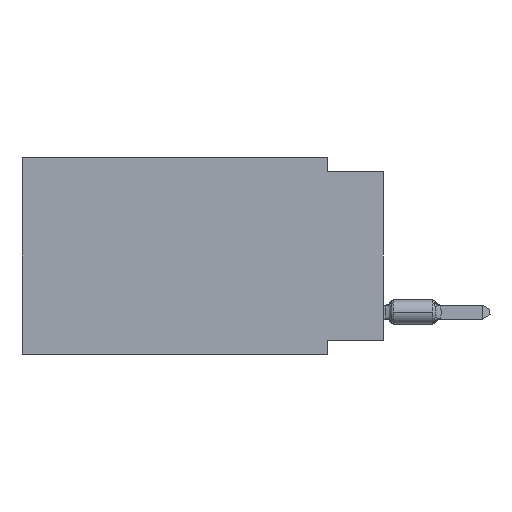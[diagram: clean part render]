
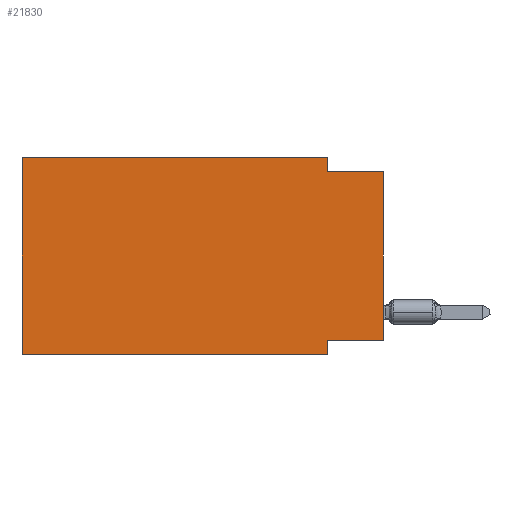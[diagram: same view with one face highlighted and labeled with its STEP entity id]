
A CAD part, left-side view. The second image highlights one B-rep face of the part: STEP entity #21830.
In plain terms, the highlighted planar face has unit normal (-1, 0, 0).
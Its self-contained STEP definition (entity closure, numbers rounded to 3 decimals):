
#452 = LINE ( 'NONE', #8074, #16340 ) ;
#2260 = EDGE_CURVE ( 'NONE', #10418, #6715, #41515, .T. ) ;
#3924 = VERTEX_POINT ( 'NONE', #22637 ) ;
#4079 = ORIENTED_EDGE ( 'NONE', *, *, #33845, .F. ) ;
#5084 = VECTOR ( 'NONE', #5566, 1000. ) ;
#5566 = DIRECTION ( 'NONE',  ( 0., 0., 1. ) ) ;
#6008 = VECTOR ( 'NONE', #10303, 1000. ) ;
#6026 = DIRECTION ( 'NONE',  ( 0., 0., -1. ) ) ;
#6108 = LINE ( 'NONE', #26974, #5084 ) ;
#6715 = VERTEX_POINT ( 'NONE', #27822 ) ;
#6781 = LINE ( 'NONE', #32423, #36512 ) ;
#7133 = ORIENTED_EDGE ( 'NONE', *, *, #13305, .F. ) ;
#8074 = CARTESIAN_POINT ( 'NONE',  ( 0., 16.383, 0. ) ) ;
#10226 = FACE_OUTER_BOUND ( 'NONE', #10283, .T. ) ;
#10283 = EDGE_LOOP ( 'NONE', ( #15879, #4079, #47292, #52221, #31678, #54057, #44423, #7133 ) ) ;
#10303 = DIRECTION ( 'NONE',  ( 0., 1., 0. ) ) ;
#10418 = VERTEX_POINT ( 'NONE', #30721 ) ;
#11754 = EDGE_CURVE ( 'NONE', #43430, #31384, #45235, .T. ) ;
#13175 = EDGE_CURVE ( 'NONE', #3924, #39061, #6108, .T. ) ;
#13305 = EDGE_CURVE ( 'NONE', #3924, #40642, #48945, .T. ) ;
#15879 = ORIENTED_EDGE ( 'NONE', *, *, #13175, .T. ) ;
#16051 = DIRECTION ( 'NONE',  ( 0., -1., 0. ) ) ;
#16340 = VECTOR ( 'NONE', #25536, 1000. ) ;
#16719 = CARTESIAN_POINT ( 'NONE',  ( 0., 2.54, 0. ) ) ;
#18103 = CARTESIAN_POINT ( 'NONE',  ( 0., 16.383, 0. ) ) ;
#18830 = EDGE_CURVE ( 'NONE', #10418, #54028, #452, .T. ) ;
#19998 = LINE ( 'NONE', #49879, #47652 ) ;
#21830 = ADVANCED_FACE ( 'NONE', ( #10226 ), #35350, .F. ) ;
#22637 = CARTESIAN_POINT ( 'NONE',  ( 0., 0., -8.255 ) ) ;
#25536 = DIRECTION ( 'NONE',  ( 0., 0., 1. ) ) ;
#25730 = DIRECTION ( 'NONE',  ( 0., 0., -1. ) ) ;
#26595 = DIRECTION ( 'NONE',  ( 1., 0., 0. ) ) ;
#26870 = VECTOR ( 'NONE', #32484, 1000. ) ;
#26974 = CARTESIAN_POINT ( 'NONE',  ( 0., 0., 0. ) ) ;
#27822 = CARTESIAN_POINT ( 'NONE',  ( 0., 2.54, -8.89 ) ) ;
#28041 = CARTESIAN_POINT ( 'NONE',  ( 0., 0., -0.635 ) ) ;
#30721 = CARTESIAN_POINT ( 'NONE',  ( 0., 16.383, -8.89 ) ) ;
#31384 = VERTEX_POINT ( 'NONE', #52134 ) ;
#31678 = ORIENTED_EDGE ( 'NONE', *, *, #18830, .F. ) ;
#32132 = DIRECTION ( 'NONE',  ( 0., 0., -1. ) ) ;
#32423 = CARTESIAN_POINT ( 'NONE',  ( 0., 2.54, -8.89 ) ) ;
#32484 = DIRECTION ( 'NONE',  ( 0., -1., 0. ) ) ;
#33845 = EDGE_CURVE ( 'NONE', #31384, #39061, #39145, .T. ) ;
#35350 = PLANE ( 'NONE',  #41763 ) ;
#36512 = VECTOR ( 'NONE', #32132, 1000. ) ;
#39061 = VERTEX_POINT ( 'NONE', #28041 ) ;
#39145 = LINE ( 'NONE', #55516, #47612 ) ;
#40512 = CARTESIAN_POINT ( 'NONE',  ( 0., 0., -8.255 ) ) ;
#40642 = VERTEX_POINT ( 'NONE', #41269 ) ;
#41269 = CARTESIAN_POINT ( 'NONE',  ( 0., 2.54, -8.255 ) ) ;
#41515 = LINE ( 'NONE', #53915, #26870 ) ;
#41763 = AXIS2_PLACEMENT_3D ( 'NONE', #53382, #26595, #6026 ) ;
#43430 = VERTEX_POINT ( 'NONE', #48754 ) ;
#44423 = ORIENTED_EDGE ( 'NONE', *, *, #50243, .F. ) ;
#45235 = LINE ( 'NONE', #16719, #45657 ) ;
#45657 = VECTOR ( 'NONE', #25730, 1000. ) ;
#47292 = ORIENTED_EDGE ( 'NONE', *, *, #11754, .F. ) ;
#47612 = VECTOR ( 'NONE', #47897, 1000. ) ;
#47652 = VECTOR ( 'NONE', #16051, 1000. ) ;
#47897 = DIRECTION ( 'NONE',  ( 0., -1., 0. ) ) ;
#48754 = CARTESIAN_POINT ( 'NONE',  ( 0., 2.54, 0. ) ) ;
#48945 = LINE ( 'NONE', #40512, #6008 ) ;
#49879 = CARTESIAN_POINT ( 'NONE',  ( 0., 16.383, 0. ) ) ;
#50243 = EDGE_CURVE ( 'NONE', #40642, #6715, #6781, .T. ) ;
#52134 = CARTESIAN_POINT ( 'NONE',  ( 0., 2.54, -0.635 ) ) ;
#52221 = ORIENTED_EDGE ( 'NONE', *, *, #55662, .F. ) ;
#53382 = CARTESIAN_POINT ( 'NONE',  ( 0., 16.383, 0. ) ) ;
#53915 = CARTESIAN_POINT ( 'NONE',  ( 0., 16.383, -8.89 ) ) ;
#54028 = VERTEX_POINT ( 'NONE', #18103 ) ;
#54057 = ORIENTED_EDGE ( 'NONE', *, *, #2260, .T. ) ;
#55516 = CARTESIAN_POINT ( 'NONE',  ( 0., 0., -0.635 ) ) ;
#55662 = EDGE_CURVE ( 'NONE', #54028, #43430, #19998, .T. ) ;
